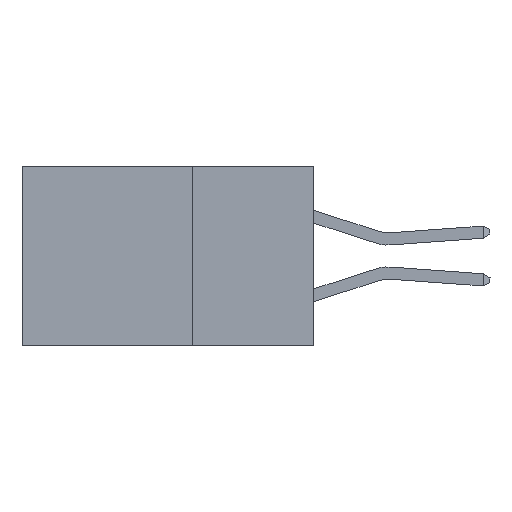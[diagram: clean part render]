
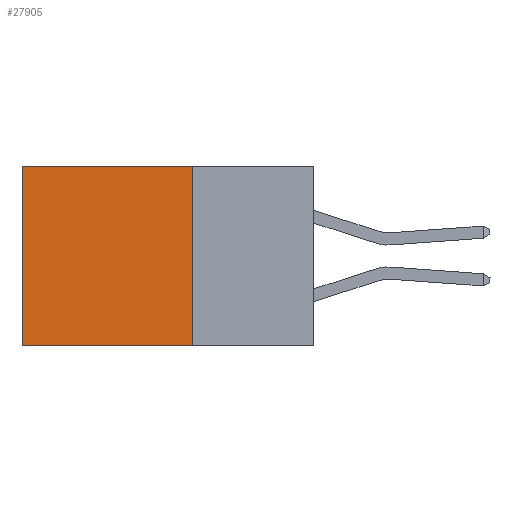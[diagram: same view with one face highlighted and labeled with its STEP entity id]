
A CAD part, left-side view. The second image highlights one B-rep face of the part: STEP entity #27905.
In plain terms, the highlighted planar face has unit normal (-1, 0, 0).
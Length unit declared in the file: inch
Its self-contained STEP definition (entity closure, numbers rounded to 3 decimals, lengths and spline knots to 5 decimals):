
#725 = DIRECTION ( 'NONE',  ( 1., 0., 0. ) ) ;
#1181 = PLANE ( 'NONE',  #29333 ) ;
#1334 = FACE_OUTER_BOUND ( 'NONE', #16332, .T. ) ;
#1871 = ORIENTED_EDGE ( 'NONE', *, *, #26165, .T. ) ;
#4489 = DIRECTION ( 'NONE',  ( 0., 0., -1. ) ) ;
#6329 = DIRECTION ( 'NONE',  ( 0., 1., 0. ) ) ;
#8379 = EDGE_CURVE ( 'NONE', #23642, #18177, #14519, .T. ) ;
#8650 = VECTOR ( 'NONE', #4489, 39.37008 ) ;
#8926 = VECTOR ( 'NONE', #17238, 39.37008 ) ;
#9360 = EDGE_CURVE ( 'NONE', #23642, #29220, #17391, .T. ) ;
#10564 = CARTESIAN_POINT ( 'NONE',  ( 0.2875, 0.25, -0.37 ) ) ;
#10791 = VECTOR ( 'NONE', #17946, 39.37008 ) ;
#10878 = DIRECTION ( 'NONE',  ( 0., 0., -1. ) ) ;
#14519 = LINE ( 'NONE', #21855, #8650 ) ;
#14630 = VECTOR ( 'NONE', #6329, 39.37008 ) ;
#15424 = CARTESIAN_POINT ( 'NONE',  ( 0.2875, 0.25, 0. ) ) ;
#16332 = EDGE_LOOP ( 'NONE', ( #1871, #24997, #23244, #20092 ) ) ;
#16482 = CARTESIAN_POINT ( 'NONE',  ( 0.2875, 0.6, -0.37 ) ) ;
#16945 = CARTESIAN_POINT ( 'NONE',  ( 0.2875, 0.6, 0. ) ) ;
#16996 = LINE ( 'NONE', #10564, #14630 ) ;
#17238 = DIRECTION ( 'NONE',  ( 0., 1., 0. ) ) ;
#17391 = LINE ( 'NONE', #24565, #8926 ) ;
#17640 = LINE ( 'NONE', #24812, #10791 ) ;
#17946 = DIRECTION ( 'NONE',  ( 0., 0., -1. ) ) ;
#18177 = VERTEX_POINT ( 'NONE', #25016 ) ;
#19480 = CARTESIAN_POINT ( 'NONE',  ( 0.2875, 0.25, 0. ) ) ;
#20092 = ORIENTED_EDGE ( 'NONE', *, *, #9360, .T. ) ;
#21855 = CARTESIAN_POINT ( 'NONE',  ( 0.2875, 0.25, 0. ) ) ;
#23244 = ORIENTED_EDGE ( 'NONE', *, *, #8379, .F. ) ;
#23642 = VERTEX_POINT ( 'NONE', #19480 ) ;
#23866 = VERTEX_POINT ( 'NONE', #16482 ) ;
#24565 = CARTESIAN_POINT ( 'NONE',  ( 0.2875, 0.25, 0. ) ) ;
#24633 = EDGE_CURVE ( 'NONE', #18177, #23866, #16996, .T. ) ;
#24812 = CARTESIAN_POINT ( 'NONE',  ( 0.2875, 0.6, 0. ) ) ;
#24997 = ORIENTED_EDGE ( 'NONE', *, *, #24633, .F. ) ;
#25016 = CARTESIAN_POINT ( 'NONE',  ( 0.2875, 0.25, -0.37 ) ) ;
#26165 = EDGE_CURVE ( 'NONE', #29220, #23866, #17640, .T. ) ;
#27905 = ADVANCED_FACE ( 'NONE', ( #1334 ), #1181, .F. ) ;
#29220 = VERTEX_POINT ( 'NONE', #16945 ) ;
#29333 = AXIS2_PLACEMENT_3D ( 'NONE', #15424, #725, #10878 ) ;
